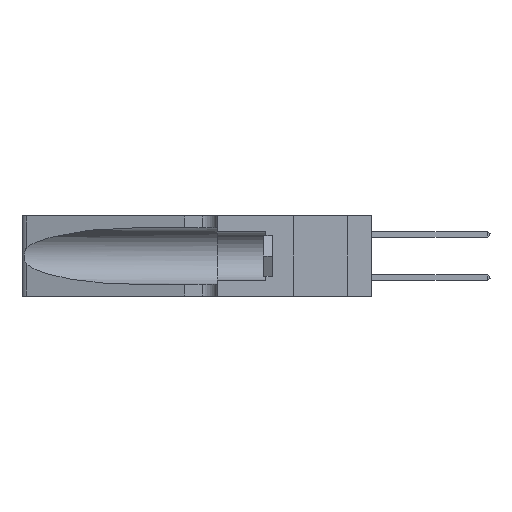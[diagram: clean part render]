
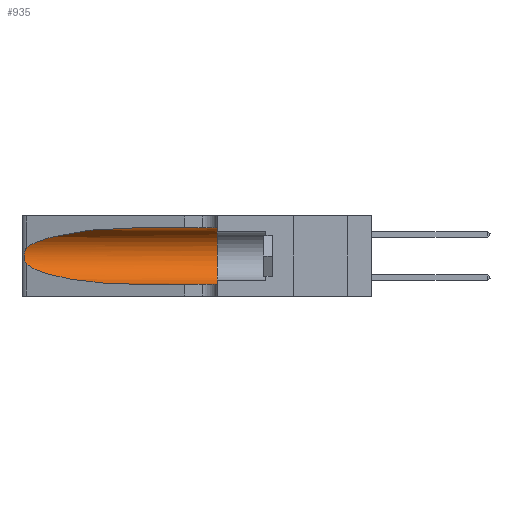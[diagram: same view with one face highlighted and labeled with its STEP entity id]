
A CAD part, left-side view. The second image highlights one B-rep face of the part: STEP entity #935.
In plain terms, the highlighted cylindrical face has radius 3.308 mm (diameter 6.617 mm), a partial arc.
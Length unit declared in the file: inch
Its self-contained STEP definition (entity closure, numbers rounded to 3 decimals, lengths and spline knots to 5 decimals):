
#80 = CARTESIAN_POINT ( 'NONE',  ( 0.25856, 1.23593, 0.16098 ) ) ;
#105 = DIRECTION ( 'NONE',  ( 0., -1., 0. ) ) ;
#935 = ADVANCED_FACE ( 'NONE', ( #2780 ), #21744, .F. ) ;
#1854 = CARTESIAN_POINT ( 'NONE',  ( 0.2373, 1.15595, 0.28018 ) ) ;
#2301 = EDGE_CURVE ( 'NONE', #25245, #24273, #23980, .T. ) ;
#2619 = CARTESIAN_POINT ( 'NONE',  ( 0.25639, 1.23186, 0.15144 ) ) ;
#2780 = FACE_OUTER_BOUND ( 'NONE', #26811, .T. ) ;
#3015 = CARTESIAN_POINT ( 'NONE',  ( 0.1305, 1.61858, 0.31525 ) ) ;
#3140 = EDGE_CURVE ( 'NONE', #13122, #14970, #12684, .T. ) ;
#3595 = CARTESIAN_POINT ( 'NONE',  ( 0.25487, 1.22718, 0.14631 ) ) ;
#3829 = AXIS2_PLACEMENT_3D ( 'NONE', #5175, #105, #22438 ) ;
#4285 = VECTOR ( 'NONE', #17874, 39.37008 ) ;
#4510 =( BOUNDED_CURVE ( )  B_SPLINE_CURVE ( 3, ( #14288, #31430, #1854, #19183 ),
 .UNSPECIFIED., .F., .F. ) 
 B_SPLINE_CURVE_WITH_KNOTS ( ( 4, 4 ),
 ( 1.5708, 2.84003 ),
 .UNSPECIFIED. ) 
 CURVE ( )  GEOMETRIC_REPRESENTATION_ITEM ( )  RATIONAL_B_SPLINE_CURVE ( ( 1., 0.87, 0.87, 1. ) ) 
 REPRESENTATION_ITEM ( '' )  );
#5046 = CARTESIAN_POINT ( 'NONE',  ( 0.25555, 1.22994, 0.2215 ) ) ;
#5152 = CARTESIAN_POINT ( 'NONE',  ( 0.25487, 1.22718, 0.14631 ) ) ;
#5175 = CARTESIAN_POINT ( 'NONE',  ( 0.1305, 1.61858, 0.185 ) ) ;
#5924 = DIRECTION ( 'NONE',  ( 0., -1., 0. ) ) ;
#6099 = CARTESIAN_POINT ( 'NONE',  ( 0.2373, 1.15595, 0.08982 ) ) ;
#6347 = LINE ( 'NONE', #18246, #19453 ) ;
#7527 = CARTESIAN_POINT ( 'NONE',  ( 0.25639, 1.23184, 0.21858 ) ) ;
#8639 = ORIENTED_EDGE ( 'NONE', *, *, #3140, .T. ) ;
#8658 = CARTESIAN_POINT ( 'NONE',  ( 0.1305, 0.35, 0.31525 ) ) ;
#8692 = EDGE_CURVE ( 'NONE', #24273, #20281, #12324, .T. ) ;
#9002 = ORIENTED_EDGE ( 'NONE', *, *, #8692, .F. ) ;
#10047 = CARTESIAN_POINT ( 'NONE',  ( 0.25854, 1.2359, 0.20912 ) ) ;
#10182 = AXIS2_PLACEMENT_3D ( 'NONE', #29145, #14481, #31621 ) ;
#11132 = CARTESIAN_POINT ( 'NONE',  ( 0.1305, 0.72297, 0.05475 ) ) ;
#11904 = ORIENTED_EDGE ( 'NONE', *, *, #20291, .T. ) ;
#12324 = CIRCLE ( 'NONE', #10182, 0.13025 ) ;
#12572 = CARTESIAN_POINT ( 'NONE',  ( 0.26075, 1.23896, 0.19203 ) ) ;
#12684 = B_SPLINE_CURVE_WITH_KNOTS ( 'NONE', 3,
 ( #22307, #5046, #7527, #24784, #10047, #27208, #12572, #29711, #15024, #80, #17490, #2619, #19912, #5152 ),
 .UNSPECIFIED., .F., .F.,
 ( 4, 2, 2, 2, 2, 2, 4 ),
 ( 0., 0.00027, 0.00053, 0.00107, 0.0016, 0.00187, 0.00214 ),
 .UNSPECIFIED. ) ;
#13122 = VERTEX_POINT ( 'NONE', #23087 ) ;
#14288 = CARTESIAN_POINT ( 'NONE',  ( 0.1305, 0.72297, 0.31525 ) ) ;
#14481 = DIRECTION ( 'NONE',  ( 0., 1., 0. ) ) ;
#14970 = VERTEX_POINT ( 'NONE', #20277 ) ;
#15024 = CARTESIAN_POINT ( 'NONE',  ( 0.26017, 1.23833, 0.17102 ) ) ;
#16660 = EDGE_CURVE ( 'NONE', #22229, #20281, #6347, .T. ) ;
#17490 = CARTESIAN_POINT ( 'NONE',  ( 0.25789, 1.23486, 0.15765 ) ) ;
#17874 = DIRECTION ( 'NONE',  ( 0., -1., 0. ) ) ;
#18246 = CARTESIAN_POINT ( 'NONE',  ( 0.1305, 1.61858, 0.05475 ) ) ;
#19183 = CARTESIAN_POINT ( 'NONE',  ( 0.25487, 1.22718, 0.22369 ) ) ;
#19453 = VECTOR ( 'NONE', #5924, 39.37008 ) ;
#19912 = CARTESIAN_POINT ( 'NONE',  ( 0.25555, 1.22993, 0.14849 ) ) ;
#20277 = CARTESIAN_POINT ( 'NONE',  ( 0.25487, 1.22718, 0.14631 ) ) ;
#20281 = VERTEX_POINT ( 'NONE', #31320 ) ;
#20291 = EDGE_CURVE ( 'NONE', #25245, #13122, #4510, .T. ) ;
#20746 = EDGE_CURVE ( 'NONE', #14970, #22229, #30763, .T. ) ;
#21410 = ORIENTED_EDGE ( 'NONE', *, *, #2301, .F. ) ;
#21509 = CARTESIAN_POINT ( 'NONE',  ( 0.1305, 0.72297, 0.31525 ) ) ;
#21744 = CYLINDRICAL_SURFACE ( 'NONE', #3829, 0.13025 ) ;
#22212 = ORIENTED_EDGE ( 'NONE', *, *, #20746, .T. ) ;
#22229 = VERTEX_POINT ( 'NONE', #27799 ) ;
#22307 = CARTESIAN_POINT ( 'NONE',  ( 0.25487, 1.22718, 0.22369 ) ) ;
#22438 = DIRECTION ( 'NONE',  ( 0., 0., -1. ) ) ;
#23087 = CARTESIAN_POINT ( 'NONE',  ( 0.25487, 1.22718, 0.22369 ) ) ;
#23980 = LINE ( 'NONE', #3015, #4285 ) ;
#24086 = ORIENTED_EDGE ( 'NONE', *, *, #16660, .T. ) ;
#24273 = VERTEX_POINT ( 'NONE', #8658 ) ;
#24784 = CARTESIAN_POINT ( 'NONE',  ( 0.25787, 1.23484, 0.2124 ) ) ;
#25245 = VERTEX_POINT ( 'NONE', #21509 ) ;
#25824 = CARTESIAN_POINT ( 'NONE',  ( 0.18966, 0.96281, 0.05475 ) ) ;
#26811 = EDGE_LOOP ( 'NONE', ( #11904, #8639, #22212, #24086, #9002, #21410 ) ) ;
#27208 = CARTESIAN_POINT ( 'NONE',  ( 0.26018, 1.23835, 0.19895 ) ) ;
#27799 = CARTESIAN_POINT ( 'NONE',  ( 0.1305, 0.72297, 0.05475 ) ) ;
#29145 = CARTESIAN_POINT ( 'NONE',  ( 0.1305, 0.35, 0.185 ) ) ;
#29711 = CARTESIAN_POINT ( 'NONE',  ( 0.26075, 1.23896, 0.178 ) ) ;
#30763 =( BOUNDED_CURVE ( )  B_SPLINE_CURVE ( 3, ( #3595, #6099, #25824, #11132 ),
 .UNSPECIFIED., .F., .F. ) 
 B_SPLINE_CURVE_WITH_KNOTS ( ( 4, 4 ),
 ( 3.44316, 4.71239 ),
 .UNSPECIFIED. ) 
 CURVE ( )  GEOMETRIC_REPRESENTATION_ITEM ( )  RATIONAL_B_SPLINE_CURVE ( ( 1., 0.87, 0.87, 1. ) ) 
 REPRESENTATION_ITEM ( '' )  );
#31320 = CARTESIAN_POINT ( 'NONE',  ( 0.1305, 0.35, 0.05475 ) ) ;
#31430 = CARTESIAN_POINT ( 'NONE',  ( 0.18966, 0.96281, 0.31525 ) ) ;
#31621 = DIRECTION ( 'NONE',  ( 0., 0., 1. ) ) ;
